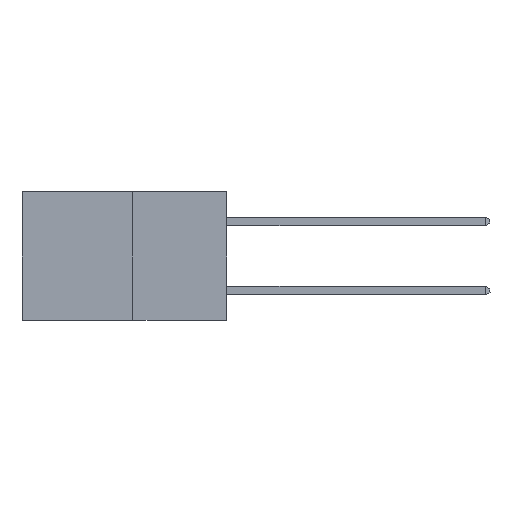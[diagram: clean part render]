
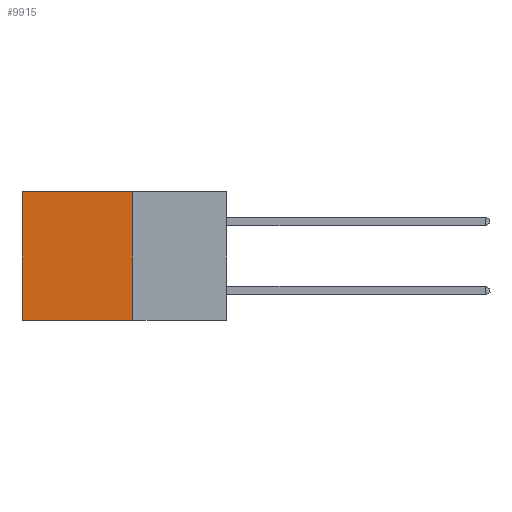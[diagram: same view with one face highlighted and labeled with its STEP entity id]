
A CAD part, left-side view. The second image highlights one B-rep face of the part: STEP entity #9915.
In plain terms, the highlighted planar face has unit normal (-1, 0, 0).
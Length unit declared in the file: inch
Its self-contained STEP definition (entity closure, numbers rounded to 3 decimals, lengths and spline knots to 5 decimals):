
#721 = VECTOR ( 'NONE', #11685, 39.37008 ) ;
#916 = VECTOR ( 'NONE', #16836, 39.37008 ) ;
#1620 = CARTESIAN_POINT ( 'NONE',  ( 0.277, 0.27, -0.37 ) ) ;
#1843 = VECTOR ( 'NONE', #9986, 39.37008 ) ;
#2199 = CARTESIAN_POINT ( 'NONE',  ( 0.277, 0.27, -0.37 ) ) ;
#3604 = ORIENTED_EDGE ( 'NONE', *, *, #16206, .F. ) ;
#3731 = DIRECTION ( 'NONE',  ( 0., 1., 0. ) ) ;
#3775 = CARTESIAN_POINT ( 'NONE',  ( 0.277, 0.59, -0.37 ) ) ;
#5207 = ORIENTED_EDGE ( 'NONE', *, *, #17119, .F. ) ;
#6439 = PLANE ( 'NONE',  #6728 ) ;
#6728 = AXIS2_PLACEMENT_3D ( 'NONE', #2199, #8468, #23060 ) ;
#7171 = ORIENTED_EDGE ( 'NONE', *, *, #16502, .T. ) ;
#7243 = VERTEX_POINT ( 'NONE', #16822 ) ;
#8468 = DIRECTION ( 'NONE',  ( 1., 0., 0. ) ) ;
#8725 = VECTOR ( 'NONE', #3731, 39.37008 ) ;
#9915 = ADVANCED_FACE ( 'NONE', ( #12723 ), #6439, .F. ) ;
#9986 = DIRECTION ( 'NONE',  ( 0., 0., -1. ) ) ;
#10278 = CARTESIAN_POINT ( 'NONE',  ( 0.277, 0.27, -0.37 ) ) ;
#11685 = DIRECTION ( 'NONE',  ( 0., 0., -1. ) ) ;
#12385 = VERTEX_POINT ( 'NONE', #18432 ) ;
#12723 = FACE_OUTER_BOUND ( 'NONE', #18791, .T. ) ;
#12946 = LINE ( 'NONE', #10278, #1843 ) ;
#13401 = CARTESIAN_POINT ( 'NONE',  ( 0.277, 0.59, 0. ) ) ;
#14717 = CARTESIAN_POINT ( 'NONE',  ( 0.277, 0.27, 0. ) ) ;
#14947 = LINE ( 'NONE', #1620, #8725 ) ;
#16206 = EDGE_CURVE ( 'NONE', #12385, #22452, #14947, .T. ) ;
#16502 = EDGE_CURVE ( 'NONE', #7243, #20878, #18206, .T. ) ;
#16822 = CARTESIAN_POINT ( 'NONE',  ( 0.277, 0.27, 0. ) ) ;
#16836 = DIRECTION ( 'NONE',  ( 0., 1., 0. ) ) ;
#17119 = EDGE_CURVE ( 'NONE', #7243, #12385, #12946, .T. ) ;
#18206 = LINE ( 'NONE', #14717, #916 ) ;
#18432 = CARTESIAN_POINT ( 'NONE',  ( 0.277, 0.27, -0.37 ) ) ;
#18791 = EDGE_LOOP ( 'NONE', ( #20859, #3604, #5207, #7171 ) ) ;
#19997 = CARTESIAN_POINT ( 'NONE',  ( 0.277, 0.59, -0.37 ) ) ;
#20859 = ORIENTED_EDGE ( 'NONE', *, *, #23081, .T. ) ;
#20878 = VERTEX_POINT ( 'NONE', #13401 ) ;
#20945 = LINE ( 'NONE', #19997, #721 ) ;
#22452 = VERTEX_POINT ( 'NONE', #3775 ) ;
#23060 = DIRECTION ( 'NONE',  ( 0., 0., -1. ) ) ;
#23081 = EDGE_CURVE ( 'NONE', #20878, #22452, #20945, .T. ) ;
